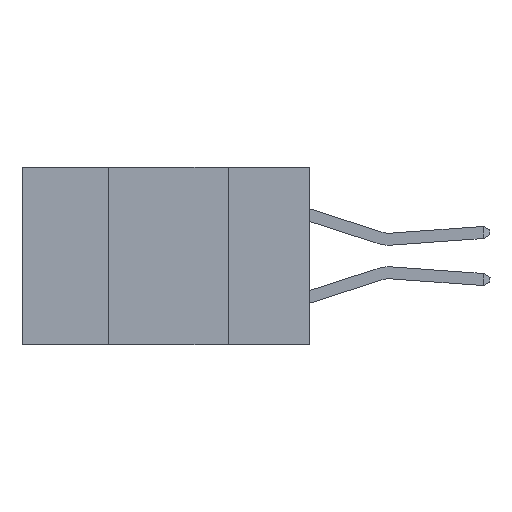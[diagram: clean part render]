
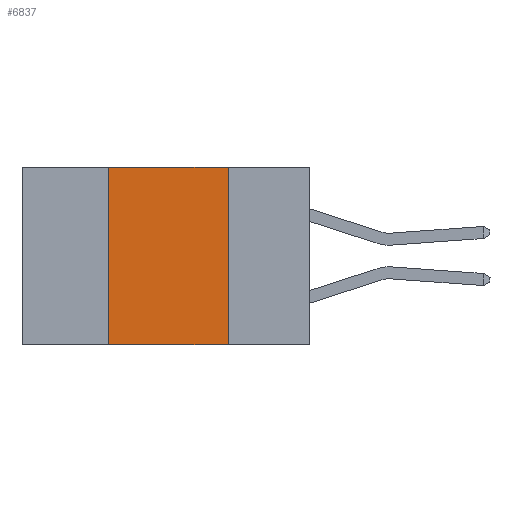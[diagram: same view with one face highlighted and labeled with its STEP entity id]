
A CAD part, left-side view. The second image highlights one B-rep face of the part: STEP entity #6837.
In plain terms, the highlighted planar face has unit normal (-1, 0, 0).
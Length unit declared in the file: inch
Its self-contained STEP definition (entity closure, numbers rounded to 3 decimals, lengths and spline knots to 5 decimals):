
#436 = EDGE_CURVE ( 'NONE', #6260, #7508, #4822, .T. ) ;
#504 = ORIENTED_EDGE ( 'NONE', *, *, #3965, .T. ) ;
#770 = DIRECTION ( 'NONE',  ( 0., -1., 0. ) ) ;
#814 = AXIS2_PLACEMENT_3D ( 'NONE', #9037, #6752, #4562 ) ;
#839 = FACE_OUTER_BOUND ( 'NONE', #1662, .T. ) ;
#1374 = VECTOR ( 'NONE', #770, 39.37008 ) ;
#1662 = EDGE_LOOP ( 'NONE', ( #7646, #5863, #8134, #504 ) ) ;
#1707 = LINE ( 'NONE', #5721, #2741 ) ;
#2418 = CARTESIAN_POINT ( 'NONE',  ( 0., 0.42, -0.37 ) ) ;
#2477 = DIRECTION ( 'NONE',  ( 0., 0., -1. ) ) ;
#2741 = VECTOR ( 'NONE', #3592, 39.37008 ) ;
#3592 = DIRECTION ( 'NONE',  ( 0., -1., 0. ) ) ;
#3618 = CARTESIAN_POINT ( 'NONE',  ( 0., 0.42, 0. ) ) ;
#3751 = EDGE_CURVE ( 'NONE', #7508, #6475, #5892, .T. ) ;
#3965 = EDGE_CURVE ( 'NONE', #6260, #4623, #1707, .T. ) ;
#4474 = EDGE_CURVE ( 'NONE', #6475, #4623, #7084, .T. ) ;
#4562 = DIRECTION ( 'NONE',  ( 0., 0., -1. ) ) ;
#4623 = VERTEX_POINT ( 'NONE', #8631 ) ;
#4813 = DIRECTION ( 'NONE',  ( 0., 0., 1. ) ) ;
#4822 = LINE ( 'NONE', #7755, #7060 ) ;
#5649 = VECTOR ( 'NONE', #2477, 39.37008 ) ;
#5721 = CARTESIAN_POINT ( 'NONE',  ( 0., 0.6, -0.37 ) ) ;
#5863 = ORIENTED_EDGE ( 'NONE', *, *, #3751, .F. ) ;
#5892 = LINE ( 'NONE', #6090, #1374 ) ;
#6090 = CARTESIAN_POINT ( 'NONE',  ( 0., 0.6, 0. ) ) ;
#6260 = VERTEX_POINT ( 'NONE', #2418 ) ;
#6475 = VERTEX_POINT ( 'NONE', #9536 ) ;
#6752 = DIRECTION ( 'NONE',  ( 1., 0., 0. ) ) ;
#6837 = ADVANCED_FACE ( 'NONE', ( #839 ), #7319, .F. ) ;
#7060 = VECTOR ( 'NONE', #4813, 39.37008 ) ;
#7084 = LINE ( 'NONE', #7458, #5649 ) ;
#7319 = PLANE ( 'NONE',  #814 ) ;
#7458 = CARTESIAN_POINT ( 'NONE',  ( 0., 0.17, 0. ) ) ;
#7508 = VERTEX_POINT ( 'NONE', #3618 ) ;
#7646 = ORIENTED_EDGE ( 'NONE', *, *, #4474, .F. ) ;
#7755 = CARTESIAN_POINT ( 'NONE',  ( 0., 0.42, 0. ) ) ;
#8134 = ORIENTED_EDGE ( 'NONE', *, *, #436, .F. ) ;
#8631 = CARTESIAN_POINT ( 'NONE',  ( 0., 0.17, -0.37 ) ) ;
#9037 = CARTESIAN_POINT ( 'NONE',  ( 0., 0.6, 0. ) ) ;
#9536 = CARTESIAN_POINT ( 'NONE',  ( 0., 0.17, 0. ) ) ;
